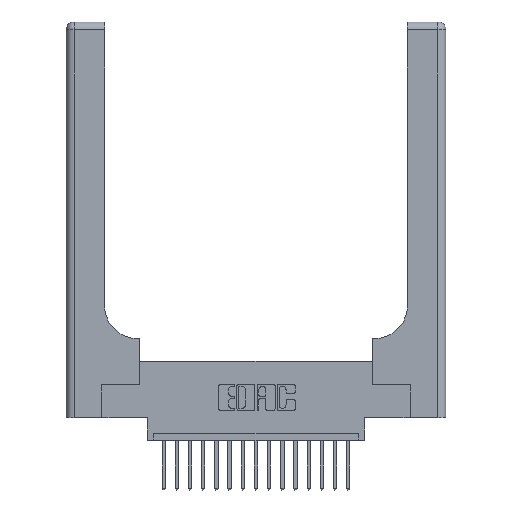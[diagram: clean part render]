
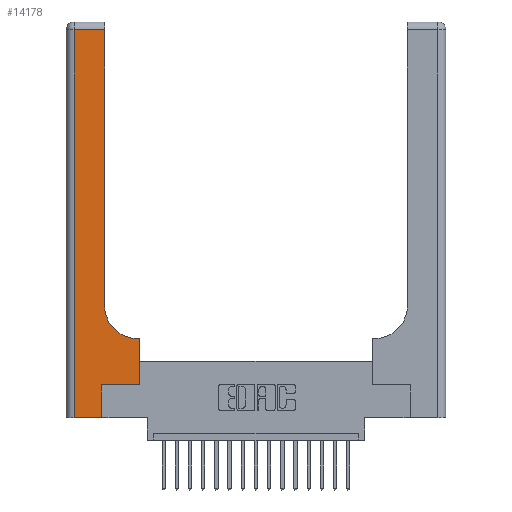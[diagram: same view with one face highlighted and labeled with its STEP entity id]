
A CAD part, top view. The second image highlights one B-rep face of the part: STEP entity #14178.
In plain terms, the highlighted planar face has unit normal (0, 0, 1).
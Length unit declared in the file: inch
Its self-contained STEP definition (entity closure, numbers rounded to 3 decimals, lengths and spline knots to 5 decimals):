
#503 = CARTESIAN_POINT ( 'NONE',  ( 0., 2.94, 0.37 ) ) ;
#684 = DIRECTION ( 'NONE',  ( 0., 0., -1. ) ) ;
#692 = VERTEX_POINT ( 'NONE', #13694 ) ;
#736 = VECTOR ( 'NONE', #15073, 39.37008 ) ;
#884 = CARTESIAN_POINT ( 'NONE',  ( 0.5585, 0.6, 0.37 ) ) ;
#1219 = EDGE_CURVE ( 'NONE', #9073, #9605, #17180, .T. ) ;
#1562 = VERTEX_POINT ( 'NONE', #9492 ) ;
#1613 = ORIENTED_EDGE ( 'NONE', *, *, #9984, .T. ) ;
#1617 = EDGE_CURVE ( 'NONE', #12092, #1562, #19123, .T. ) ;
#1772 = VECTOR ( 'NONE', #14883, 39.37008 ) ;
#2054 = EDGE_CURVE ( 'NONE', #4759, #3761, #5397, .T. ) ;
#2386 = DIRECTION ( 'NONE',  ( 0., 1., 0. ) ) ;
#2558 = DIRECTION ( 'NONE',  ( 1., 0., 0. ) ) ;
#2706 = CARTESIAN_POINT ( 'NONE',  ( 0.5415, 0.85, 0.37 ) ) ;
#3029 = CARTESIAN_POINT ( 'NONE',  ( 0.269, 0., 0.37 ) ) ;
#3069 = VERTEX_POINT ( 'NONE', #884 ) ;
#3502 = CARTESIAN_POINT ( 'NONE',  ( 0.2915, 0.85, 0.37 ) ) ;
#3761 = VERTEX_POINT ( 'NONE', #18947 ) ;
#3983 = CARTESIAN_POINT ( 'NONE',  ( 0.2915, 2.94, 0.37 ) ) ;
#4080 = VECTOR ( 'NONE', #2386, 39.37008 ) ;
#4163 = LINE ( 'NONE', #17105, #12001 ) ;
#4523 = DIRECTION ( 'NONE',  ( -1., 0., 0. ) ) ;
#4759 = VERTEX_POINT ( 'NONE', #3029 ) ;
#4844 = CARTESIAN_POINT ( 'NONE',  ( 0.06, 3., 0.37 ) ) ;
#5242 = CARTESIAN_POINT ( 'NONE',  ( 0.5415, 0.6, 0.37 ) ) ;
#5366 = VECTOR ( 'NONE', #11117, 39.37008 ) ;
#5396 = ORIENTED_EDGE ( 'NONE', *, *, #16631, .T. ) ;
#5397 = LINE ( 'NONE', #12074, #736 ) ;
#5465 = AXIS2_PLACEMENT_3D ( 'NONE', #2706, #11951, #2558 ) ;
#6478 = LINE ( 'NONE', #10810, #19431 ) ;
#6527 = VERTEX_POINT ( 'NONE', #14063 ) ;
#7000 = PLANE ( 'NONE',  #13248 ) ;
#7416 = ORIENTED_EDGE ( 'NONE', *, *, #1617, .T. ) ;
#7905 = EDGE_LOOP ( 'NONE', ( #1613, #7416, #19540, #12109, #18715, #12454, #5396, #10007, #13837 ) ) ;
#8236 = EDGE_CURVE ( 'NONE', #3761, #6527, #6478, .T. ) ;
#8628 = EDGE_CURVE ( 'NONE', #692, #4759, #10109, .T. ) ;
#9073 = VERTEX_POINT ( 'NONE', #5242 ) ;
#9130 = VECTOR ( 'NONE', #12811, 39.37008 ) ;
#9267 = DIRECTION ( 'NONE',  ( 1., 0., 0. ) ) ;
#9492 = CARTESIAN_POINT ( 'NONE',  ( 0.06, 2.94, 0.37 ) ) ;
#9605 = VERTEX_POINT ( 'NONE', #3502 ) ;
#9984 = EDGE_CURVE ( 'NONE', #9605, #12092, #4163, .T. ) ;
#10007 = ORIENTED_EDGE ( 'NONE', *, *, #10024, .T. ) ;
#10024 = EDGE_CURVE ( 'NONE', #3069, #9073, #19840, .T. ) ;
#10109 = LINE ( 'NONE', #14818, #1772 ) ;
#10810 = CARTESIAN_POINT ( 'NONE',  ( 0.269, 0.25, 0.37 ) ) ;
#11117 = DIRECTION ( 'NONE',  ( 0., -1., 0. ) ) ;
#11536 = EDGE_CURVE ( 'NONE', #1562, #692, #17829, .T. ) ;
#11606 = DIRECTION ( 'NONE',  ( -1., 0., 0. ) ) ;
#11774 = CARTESIAN_POINT ( 'NONE',  ( 0.5585, 0.25, 0.37 ) ) ;
#11918 = LINE ( 'NONE', #11774, #4080 ) ;
#11951 = DIRECTION ( 'NONE',  ( 0., 0., -1. ) ) ;
#12001 = VECTOR ( 'NONE', #13890, 39.37008 ) ;
#12074 = CARTESIAN_POINT ( 'NONE',  ( 0.269, 0., 0.37 ) ) ;
#12092 = VERTEX_POINT ( 'NONE', #3983 ) ;
#12109 = ORIENTED_EDGE ( 'NONE', *, *, #8628, .T. ) ;
#12245 = VECTOR ( 'NONE', #4523, 39.37008 ) ;
#12454 = ORIENTED_EDGE ( 'NONE', *, *, #8236, .T. ) ;
#12811 = DIRECTION ( 'NONE',  ( -1., 0., 0. ) ) ;
#13248 = AXIS2_PLACEMENT_3D ( 'NONE', #16324, #684, #11606 ) ;
#13694 = CARTESIAN_POINT ( 'NONE',  ( 0.06, 0., 0.37 ) ) ;
#13837 = ORIENTED_EDGE ( 'NONE', *, *, #1219, .T. ) ;
#13890 = DIRECTION ( 'NONE',  ( 0., 1., 0. ) ) ;
#14063 = CARTESIAN_POINT ( 'NONE',  ( 0.5585, 0.25, 0.37 ) ) ;
#14178 = ADVANCED_FACE ( 'NONE', ( #19128 ), #7000, .F. ) ;
#14818 = CARTESIAN_POINT ( 'NONE',  ( 0., 0., 0.37 ) ) ;
#14883 = DIRECTION ( 'NONE',  ( 1., 0., 0. ) ) ;
#15073 = DIRECTION ( 'NONE',  ( 0., 1., 0. ) ) ;
#16324 = CARTESIAN_POINT ( 'NONE',  ( 0., 3., 0.37 ) ) ;
#16631 = EDGE_CURVE ( 'NONE', #6527, #3069, #11918, .T. ) ;
#17105 = CARTESIAN_POINT ( 'NONE',  ( 0.2915, 3., 0.37 ) ) ;
#17180 = CIRCLE ( 'NONE', #5465, 0.25 ) ;
#17829 = LINE ( 'NONE', #4844, #5366 ) ;
#18715 = ORIENTED_EDGE ( 'NONE', *, *, #2054, .T. ) ;
#18947 = CARTESIAN_POINT ( 'NONE',  ( 0.269, 0.25, 0.37 ) ) ;
#19123 = LINE ( 'NONE', #503, #9130 ) ;
#19128 = FACE_OUTER_BOUND ( 'NONE', #7905, .T. ) ;
#19431 = VECTOR ( 'NONE', #9267, 39.37008 ) ;
#19540 = ORIENTED_EDGE ( 'NONE', *, *, #11536, .T. ) ;
#19840 = LINE ( 'NONE', #20265, #12245 ) ;
#20265 = CARTESIAN_POINT ( 'NONE',  ( 0.2915, 0.6, 0.37 ) ) ;
